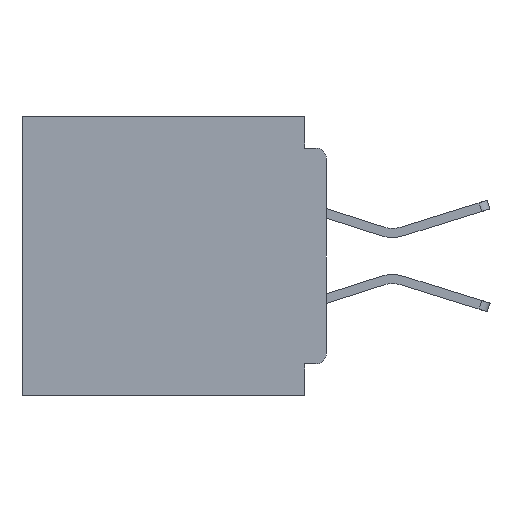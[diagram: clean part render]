
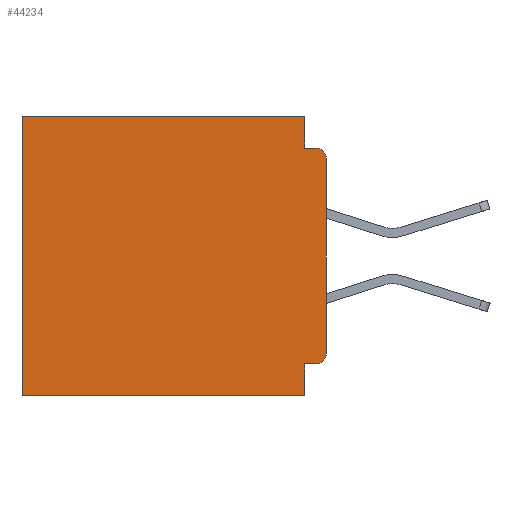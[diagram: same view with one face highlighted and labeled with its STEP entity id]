
A CAD part, left-side view. The second image highlights one B-rep face of the part: STEP entity #44234.
In plain terms, the highlighted planar face has unit normal (-1, 0, 0).
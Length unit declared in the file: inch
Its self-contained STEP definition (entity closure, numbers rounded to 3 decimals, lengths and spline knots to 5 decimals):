
#1244 = EDGE_CURVE ( 'NONE', #22756, #47502, #56998, .T. ) ;
#2204 = EDGE_LOOP ( 'NONE', ( #27140, #55624, #23377, #24893, #18044, #27202, #2755, #57187, #48969, #11984 ) ) ;
#2272 = CARTESIAN_POINT ( 'NONE',  ( 0.3, 0., -0.4 ) ) ;
#2735 = DIRECTION ( 'NONE',  ( 0., 0., -1. ) ) ;
#2755 = ORIENTED_EDGE ( 'NONE', *, *, #16958, .F. ) ;
#4473 = EDGE_CURVE ( 'NONE', #50835, #56271, #22916, .T. ) ;
#4743 = VERTEX_POINT ( 'NONE', #47882 ) ;
#5026 = LINE ( 'NONE', #2272, #27926 ) ;
#5313 = CARTESIAN_POINT ( 'NONE',  ( 0.3, 0.437, -0.4 ) ) ;
#5492 = DIRECTION ( 'NONE',  ( 0., 1., 0. ) ) ;
#6268 = EDGE_CURVE ( 'NONE', #59376, #42692, #57291, .T. ) ;
#7192 = CARTESIAN_POINT ( 'NONE',  ( 0.3, 0.437, 0. ) ) ;
#8993 = CIRCLE ( 'NONE', #60706, 0.015 ) ;
#10067 = VECTOR ( 'NONE', #2735, 39.37008 ) ;
#11984 = ORIENTED_EDGE ( 'NONE', *, *, #59902, .T. ) ;
#12207 = EDGE_CURVE ( 'NONE', #50198, #22756, #38357, .T. ) ;
#13295 = DIRECTION ( 'NONE',  ( 0., 0., -1. ) ) ;
#13583 = CARTESIAN_POINT ( 'NONE',  ( 0.3, 0.015, -0.06 ) ) ;
#13710 = DIRECTION ( 'NONE',  ( 0., 0., -1. ) ) ;
#16221 = DIRECTION ( 'NONE',  ( 0., 1., 0. ) ) ;
#16958 = EDGE_CURVE ( 'NONE', #47502, #59183, #5026, .T. ) ;
#17432 = FACE_OUTER_BOUND ( 'NONE', #2204, .T. ) ;
#18044 = ORIENTED_EDGE ( 'NONE', *, *, #4473, .T. ) ;
#18469 = DIRECTION ( 'NONE',  ( 0., 0., -1. ) ) ;
#18629 = VECTOR ( 'NONE', #44742, 39.37008 ) ;
#20185 = CARTESIAN_POINT ( 'NONE',  ( 0.3, 0.015, -0.34 ) ) ;
#21958 = DIRECTION ( 'NONE',  ( 0., 1., 0. ) ) ;
#22212 = CARTESIAN_POINT ( 'NONE',  ( 0.3, 0.031, 0. ) ) ;
#22756 = VERTEX_POINT ( 'NONE', #33169 ) ;
#22916 = LINE ( 'NONE', #58781, #34220 ) ;
#23051 = LINE ( 'NONE', #22212, #10067 ) ;
#23377 = ORIENTED_EDGE ( 'NONE', *, *, #28330, .F. ) ;
#24893 = ORIENTED_EDGE ( 'NONE', *, *, #50071, .F. ) ;
#25100 = DIRECTION ( 'NONE',  ( 0., 0., -1. ) ) ;
#26380 = DIRECTION ( 'NONE',  ( 0., 0., -1. ) ) ;
#27099 = VECTOR ( 'NONE', #16221, 39.37008 ) ;
#27140 = ORIENTED_EDGE ( 'NONE', *, *, #6268, .F. ) ;
#27202 = ORIENTED_EDGE ( 'NONE', *, *, #35519, .T. ) ;
#27599 = CARTESIAN_POINT ( 'NONE',  ( 0.3, 0., -0.34 ) ) ;
#27926 = VECTOR ( 'NONE', #21958, 39.37008 ) ;
#28330 = EDGE_CURVE ( 'NONE', #29267, #4743, #33565, .T. ) ;
#29267 = VERTEX_POINT ( 'NONE', #40015 ) ;
#29463 = CIRCLE ( 'NONE', #36302, 0.015 ) ;
#33169 = CARTESIAN_POINT ( 'NONE',  ( 0.3, 0.031, -0.355 ) ) ;
#33565 = LINE ( 'NONE', #51844, #41792 ) ;
#34220 = VECTOR ( 'NONE', #5492, 39.37008 ) ;
#34335 = CARTESIAN_POINT ( 'NONE',  ( 0.3, 0.031, -0.4 ) ) ;
#34855 = VECTOR ( 'NONE', #13295, 39.37008 ) ;
#35187 = LINE ( 'NONE', #40434, #46416 ) ;
#35473 = CARTESIAN_POINT ( 'NONE',  ( 0.3, 0., -0.06 ) ) ;
#35519 = EDGE_CURVE ( 'NONE', #56271, #59183, #35187, .T. ) ;
#36302 = AXIS2_PLACEMENT_3D ( 'NONE', #13583, #47328, #18469 ) ;
#37991 = CARTESIAN_POINT ( 'NONE',  ( 0.3, 0.031, -0.4 ) ) ;
#38357 = LINE ( 'NONE', #45107, #27099 ) ;
#38746 = CARTESIAN_POINT ( 'NONE',  ( 0.3, 0.031, 0. ) ) ;
#40015 = CARTESIAN_POINT ( 'NONE',  ( 0.3, 0.031, -0.045 ) ) ;
#40434 = CARTESIAN_POINT ( 'NONE',  ( 0.3, 0.437, -0.4 ) ) ;
#41792 = VECTOR ( 'NONE', #61445, 39.37008 ) ;
#42216 = CARTESIAN_POINT ( 'NONE',  ( 0.3, 0., -0.4 ) ) ;
#42640 = DIRECTION ( 'NONE',  ( 1., 0., 0. ) ) ;
#42692 = VERTEX_POINT ( 'NONE', #27599 ) ;
#44234 = ADVANCED_FACE ( 'NONE', ( #17432 ), #52050, .F. ) ;
#44742 = DIRECTION ( 'NONE',  ( 0., 0., -1. ) ) ;
#45107 = CARTESIAN_POINT ( 'NONE',  ( 0.3, 0., -0.355 ) ) ;
#45422 = EDGE_CURVE ( 'NONE', #59376, #4743, #29463, .T. ) ;
#46416 = VECTOR ( 'NONE', #26380, 39.37008 ) ;
#47192 = CARTESIAN_POINT ( 'NONE',  ( 0.3, 0.015, -0.355 ) ) ;
#47328 = DIRECTION ( 'NONE',  ( -1., 0., 0. ) ) ;
#47502 = VERTEX_POINT ( 'NONE', #37991 ) ;
#47882 = CARTESIAN_POINT ( 'NONE',  ( 0.3, 0.015, -0.045 ) ) ;
#48969 = ORIENTED_EDGE ( 'NONE', *, *, #12207, .F. ) ;
#50071 = EDGE_CURVE ( 'NONE', #50835, #29267, #23051, .T. ) ;
#50198 = VERTEX_POINT ( 'NONE', #47192 ) ;
#50835 = VERTEX_POINT ( 'NONE', #38746 ) ;
#51844 = CARTESIAN_POINT ( 'NONE',  ( 0.3, 0., -0.045 ) ) ;
#52050 = PLANE ( 'NONE',  #57093 ) ;
#53828 = DIRECTION ( 'NONE',  ( -1., 0., 0. ) ) ;
#55624 = ORIENTED_EDGE ( 'NONE', *, *, #45422, .T. ) ;
#56271 = VERTEX_POINT ( 'NONE', #7192 ) ;
#56998 = LINE ( 'NONE', #34335, #18629 ) ;
#57093 = AXIS2_PLACEMENT_3D ( 'NONE', #61640, #42640, #13710 ) ;
#57187 = ORIENTED_EDGE ( 'NONE', *, *, #1244, .F. ) ;
#57291 = LINE ( 'NONE', #42216, #34855 ) ;
#58781 = CARTESIAN_POINT ( 'NONE',  ( 0.3, 0., 0. ) ) ;
#59183 = VERTEX_POINT ( 'NONE', #5313 ) ;
#59376 = VERTEX_POINT ( 'NONE', #35473 ) ;
#59902 = EDGE_CURVE ( 'NONE', #50198, #42692, #8993, .T. ) ;
#60706 = AXIS2_PLACEMENT_3D ( 'NONE', #20185, #53828, #25100 ) ;
#61445 = DIRECTION ( 'NONE',  ( 0., -1., 0. ) ) ;
#61640 = CARTESIAN_POINT ( 'NONE',  ( 0.3, 0., -0.4 ) ) ;
